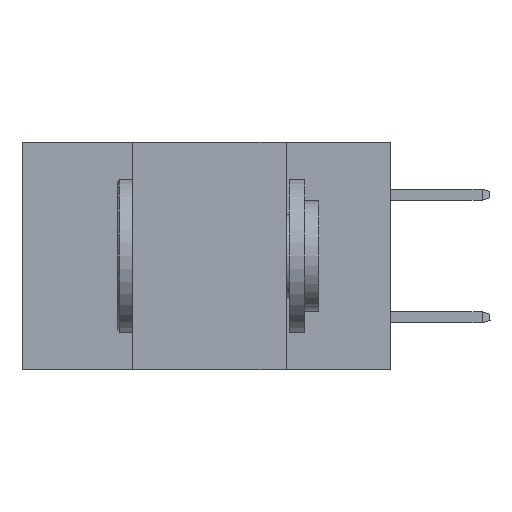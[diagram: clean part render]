
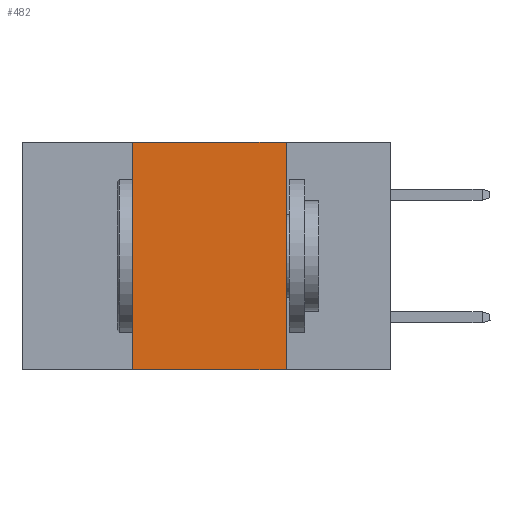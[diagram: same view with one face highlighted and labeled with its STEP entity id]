
A CAD part, left-side view. The second image highlights one B-rep face of the part: STEP entity #482.
In plain terms, the highlighted planar face has unit normal (-1, 0, 0).
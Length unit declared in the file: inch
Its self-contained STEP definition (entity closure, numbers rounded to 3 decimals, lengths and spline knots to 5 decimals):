
#482 = ADVANCED_FACE ( 'NONE', ( #6488 ), #4171, .F. ) ;
#571 = CARTESIAN_POINT ( 'NONE',  ( 0., 0.17, 0. ) ) ;
#672 = CARTESIAN_POINT ( 'NONE',  ( 0., 0.17, -0.37 ) ) ;
#1520 = ORIENTED_EDGE ( 'NONE', *, *, #6785, .F. ) ;
#1589 = ORIENTED_EDGE ( 'NONE', *, *, #8236, .F. ) ;
#1618 = ORIENTED_EDGE ( 'NONE', *, *, #13447, .F. ) ;
#1727 = CARTESIAN_POINT ( 'NONE',  ( 0., 0.42, 0. ) ) ;
#1765 = ORIENTED_EDGE ( 'NONE', *, *, #3275, .T. ) ;
#1978 = DIRECTION ( 'NONE',  ( 0., -1., 0. ) ) ;
#3135 = CARTESIAN_POINT ( 'NONE',  ( 0., 0.6, 0. ) ) ;
#3275 = EDGE_CURVE ( 'NONE', #7916, #12964, #12852, .T. ) ;
#3446 = DIRECTION ( 'NONE',  ( 0., 0., -1. ) ) ;
#3477 = DIRECTION ( 'NONE',  ( 1., 0., 0. ) ) ;
#3950 = CARTESIAN_POINT ( 'NONE',  ( 0., 0.6, -0.37 ) ) ;
#3964 = DIRECTION ( 'NONE',  ( 0., 0., 1. ) ) ;
#4171 = PLANE ( 'NONE',  #8364 ) ;
#4321 = CARTESIAN_POINT ( 'NONE',  ( 0., 0.6, 0. ) ) ;
#4728 = VECTOR ( 'NONE', #7192, 39.37008 ) ;
#5679 = CARTESIAN_POINT ( 'NONE',  ( 0., 0.17, 0. ) ) ;
#5842 = LINE ( 'NONE', #3135, #10877 ) ;
#5888 = CARTESIAN_POINT ( 'NONE',  ( 0., 0.42, -0.37 ) ) ;
#6488 = FACE_OUTER_BOUND ( 'NONE', #7637, .T. ) ;
#6785 = EDGE_CURVE ( 'NONE', #13262, #12964, #12792, .T. ) ;
#7192 = DIRECTION ( 'NONE',  ( 0., 0., -1. ) ) ;
#7583 = LINE ( 'NONE', #13125, #12582 ) ;
#7637 = EDGE_LOOP ( 'NONE', ( #1520, #1589, #1618, #1765 ) ) ;
#7852 = VECTOR ( 'NONE', #10649, 39.37008 ) ;
#7916 = VERTEX_POINT ( 'NONE', #5888 ) ;
#8236 = EDGE_CURVE ( 'NONE', #11335, #13262, #5842, .T. ) ;
#8364 = AXIS2_PLACEMENT_3D ( 'NONE', #4321, #3477, #3446 ) ;
#10649 = DIRECTION ( 'NONE',  ( 0., -1., 0. ) ) ;
#10877 = VECTOR ( 'NONE', #1978, 39.37008 ) ;
#11335 = VERTEX_POINT ( 'NONE', #1727 ) ;
#12582 = VECTOR ( 'NONE', #3964, 39.37008 ) ;
#12792 = LINE ( 'NONE', #571, #4728 ) ;
#12852 = LINE ( 'NONE', #3950, #7852 ) ;
#12964 = VERTEX_POINT ( 'NONE', #672 ) ;
#13125 = CARTESIAN_POINT ( 'NONE',  ( 0., 0.42, 0. ) ) ;
#13262 = VERTEX_POINT ( 'NONE', #5679 ) ;
#13447 = EDGE_CURVE ( 'NONE', #7916, #11335, #7583, .T. ) ;
